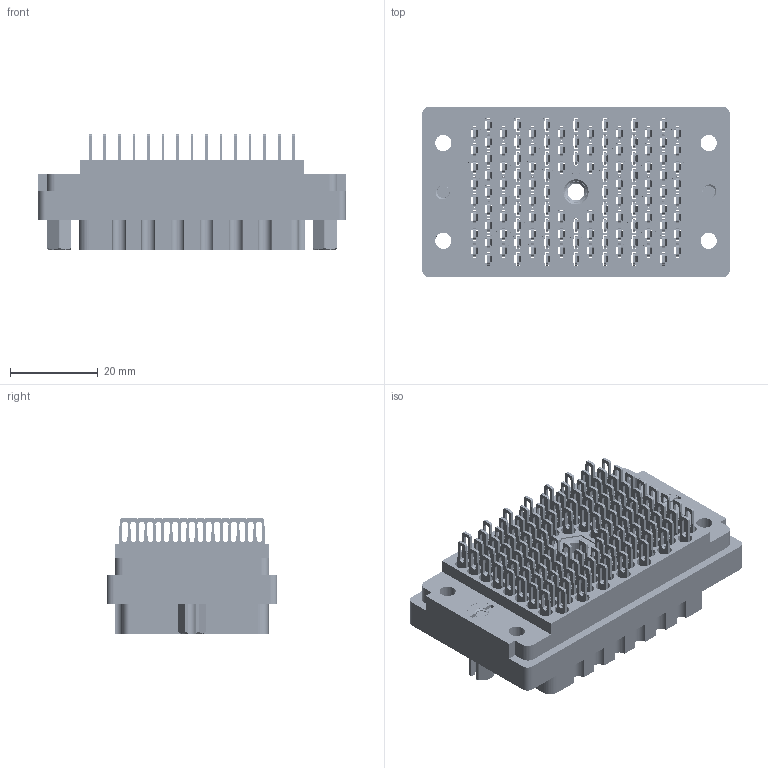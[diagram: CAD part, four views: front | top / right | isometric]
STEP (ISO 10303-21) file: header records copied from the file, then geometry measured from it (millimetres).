
FILE_DESCRIPTION (( 'STEP AP203' ), '1' );
FILE_NAME ('516-120-500-402.STEP', '2020-03-07T00:43:00', ( '' ), ( '' ), 'SwSTEP 2.0', 'SolidWorks 2016', '' );
FILE_SCHEMA (( 'CONFIG_CONTROL_DESIGN' ));
Length unit declared in the file: inch
Products named in the file (7): 516-120-500-402; 516-221-090-102_091; 516-221-090-102_090; 516 Part Receptacle_120; 516-292-001_500 Contact; 516-252-095-100; 516-252-091-102
Assembly tree (126 placements, depth 2):
  516-120-500-402
    516 Part Receptacle_120
    516-292-001_500 Contact  x120
    516-252-091-102  x2
    516-221-090-102_090
    516-252-095-100
    516-221-090-102_091
Bounding box: 69.85 x 38.73 x 26.21 mm (x, y, z)
Volume: 29754.7 mm3; surface area: 61073.8 mm2
Topology: 126 solids, 126 shells, 11813 faces, 34353 edges, 22809 vertices
Faces by surface type: plane 7008, cylinder 4011, bspline 748, cone 46
Entity records: 103796 total; most frequent: CARTESIAN_POINT 24211, ORIENTED_EDGE 16182, DIRECTION 15580, EDGE_CURVE 8091, LINE 5820, VECTOR 5820, VERTEX_POINT 5383, AXIS2_PLACEMENT_3D 4880
